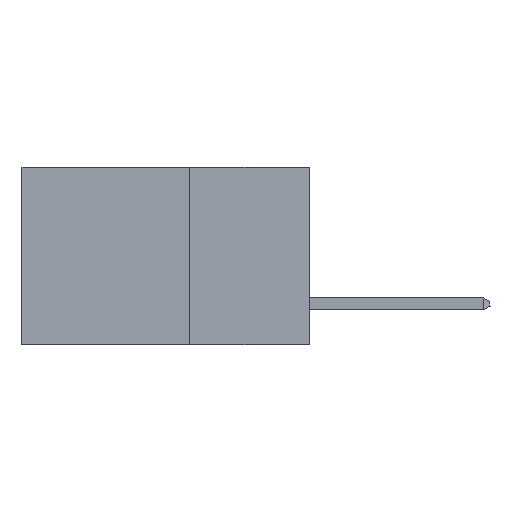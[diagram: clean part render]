
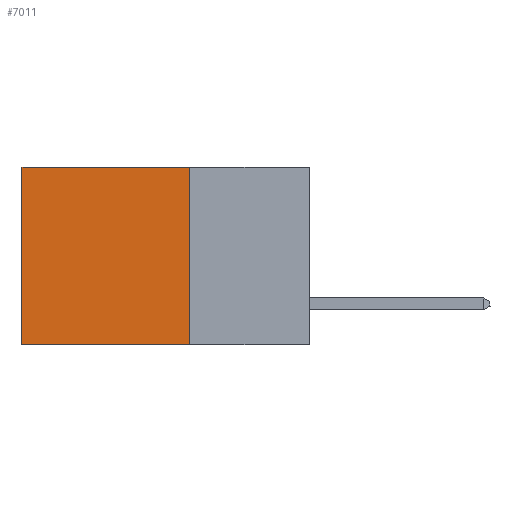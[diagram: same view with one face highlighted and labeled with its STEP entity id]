
A CAD part, left-side view. The second image highlights one B-rep face of the part: STEP entity #7011.
In plain terms, the highlighted planar face has unit normal (-1, 0, 0).
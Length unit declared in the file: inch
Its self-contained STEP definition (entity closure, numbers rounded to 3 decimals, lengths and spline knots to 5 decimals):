
#434 = VECTOR ( 'NONE', #10769, 39.37008 ) ;
#1187 = ORIENTED_EDGE ( 'NONE', *, *, #10485, .F. ) ;
#1252 = FACE_OUTER_BOUND ( 'NONE', #1265, .T. ) ;
#1265 = EDGE_LOOP ( 'NONE', ( #11158, #7623, #1187, #1594 ) ) ;
#1594 = ORIENTED_EDGE ( 'NONE', *, *, #11637, .T. ) ;
#1817 = DIRECTION ( 'NONE',  ( 1., 0., 0. ) ) ;
#2154 = EDGE_CURVE ( 'NONE', #3686, #8054, #8340, .T. ) ;
#3413 = DIRECTION ( 'NONE',  ( 0., 0., -1. ) ) ;
#3686 = VERTEX_POINT ( 'NONE', #14570 ) ;
#4087 = LINE ( 'NONE', #11603, #13916 ) ;
#4769 = VERTEX_POINT ( 'NONE', #11692 ) ;
#5376 = DIRECTION ( 'NONE',  ( 0., 1., 0. ) ) ;
#6184 = PLANE ( 'NONE',  #14107 ) ;
#6459 = CARTESIAN_POINT ( 'NONE',  ( 0.2875, 0.6, 0. ) ) ;
#6675 = DIRECTION ( 'NONE',  ( 0., 0., -1. ) ) ;
#6950 = CARTESIAN_POINT ( 'NONE',  ( 0.2875, 0.6, -0.37 ) ) ;
#7011 = ADVANCED_FACE ( 'NONE', ( #1252 ), #6184, .F. ) ;
#7596 = EDGE_CURVE ( 'NONE', #9604, #8054, #14315, .T. ) ;
#7623 = ORIENTED_EDGE ( 'NONE', *, *, #2154, .F. ) ;
#8054 = VERTEX_POINT ( 'NONE', #6950 ) ;
#8340 = LINE ( 'NONE', #13263, #15564 ) ;
#9604 = VERTEX_POINT ( 'NONE', #6459 ) ;
#10485 = EDGE_CURVE ( 'NONE', #4769, #3686, #11817, .T. ) ;
#10769 = DIRECTION ( 'NONE',  ( 0., 0., -1. ) ) ;
#11116 = CARTESIAN_POINT ( 'NONE',  ( 0.2875, 0.25, 0. ) ) ;
#11158 = ORIENTED_EDGE ( 'NONE', *, *, #7596, .T. ) ;
#11603 = CARTESIAN_POINT ( 'NONE',  ( 0.2875, 0.25, 0. ) ) ;
#11637 = EDGE_CURVE ( 'NONE', #4769, #9604, #4087, .T. ) ;
#11692 = CARTESIAN_POINT ( 'NONE',  ( 0.2875, 0.25, 0. ) ) ;
#11817 = LINE ( 'NONE', #12126, #14921 ) ;
#12126 = CARTESIAN_POINT ( 'NONE',  ( 0.2875, 0.25, 0. ) ) ;
#13263 = CARTESIAN_POINT ( 'NONE',  ( 0.2875, 0.25, -0.37 ) ) ;
#13916 = VECTOR ( 'NONE', #14922, 39.37008 ) ;
#14107 = AXIS2_PLACEMENT_3D ( 'NONE', #11116, #1817, #6675 ) ;
#14315 = LINE ( 'NONE', #14557, #434 ) ;
#14557 = CARTESIAN_POINT ( 'NONE',  ( 0.2875, 0.6, 0. ) ) ;
#14570 = CARTESIAN_POINT ( 'NONE',  ( 0.2875, 0.25, -0.37 ) ) ;
#14921 = VECTOR ( 'NONE', #3413, 39.37008 ) ;
#14922 = DIRECTION ( 'NONE',  ( 0., 1., 0. ) ) ;
#15564 = VECTOR ( 'NONE', #5376, 39.37008 ) ;
